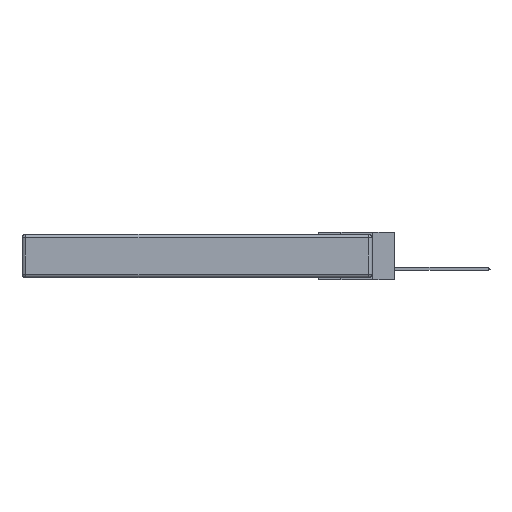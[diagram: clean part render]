
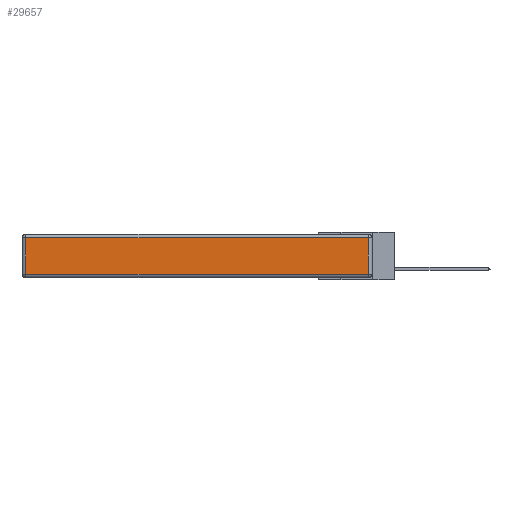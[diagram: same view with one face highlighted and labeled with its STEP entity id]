
A CAD part, left-side view. The second image highlights one B-rep face of the part: STEP entity #29657.
In plain terms, the highlighted planar face has unit normal (-1, 0, 0).
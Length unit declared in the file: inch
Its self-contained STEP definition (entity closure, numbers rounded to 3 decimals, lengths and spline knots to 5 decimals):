
#355 = ORIENTED_EDGE ( 'NONE', *, *, #27498, .T. ) ;
#1030 = FACE_OUTER_BOUND ( 'NONE', #28747, .T. ) ;
#1321 = CARTESIAN_POINT ( 'NONE',  ( 0., 0., -0.313 ) ) ;
#1453 = DIRECTION ( 'NONE',  ( -1., 0., 0. ) ) ;
#3371 = AXIS2_PLACEMENT_3D ( 'NONE', #3744, #1453, #3853 ) ;
#3744 = CARTESIAN_POINT ( 'NONE',  ( 0., 0., -0.343 ) ) ;
#3853 = DIRECTION ( 'NONE',  ( 0., 0., 1. ) ) ;
#5973 = CARTESIAN_POINT ( 'NONE',  ( 0., 0.03, -0.03 ) ) ;
#7450 = VERTEX_POINT ( 'NONE', #26897 ) ;
#8396 = VERTEX_POINT ( 'NONE', #5973 ) ;
#8527 = DIRECTION ( 'NONE',  ( 0., -1., 0. ) ) ;
#8726 = VERTEX_POINT ( 'NONE', #10129 ) ;
#9781 = LINE ( 'NONE', #1321, #25266 ) ;
#10129 = CARTESIAN_POINT ( 'NONE',  ( 0., 0.03, -0.313 ) ) ;
#10748 = CARTESIAN_POINT ( 'NONE',  ( 0., 2.72, -0.343 ) ) ;
#10846 = LINE ( 'NONE', #10748, #16578 ) ;
#12930 = PLANE ( 'NONE',  #3371 ) ;
#13310 = LINE ( 'NONE', #17860, #27780 ) ;
#15014 = ORIENTED_EDGE ( 'NONE', *, *, #17066, .T. ) ;
#15213 = CARTESIAN_POINT ( 'NONE',  ( 0., 2.72, -0.313 ) ) ;
#16578 = VECTOR ( 'NONE', #29618, 39.37008 ) ;
#17066 = EDGE_CURVE ( 'NONE', #7450, #24950, #10846, .T. ) ;
#17439 = ORIENTED_EDGE ( 'NONE', *, *, #23366, .T. ) ;
#17860 = CARTESIAN_POINT ( 'NONE',  ( 0., 0.03, -0.343 ) ) ;
#19138 = VECTOR ( 'NONE', #21898, 39.37008 ) ;
#19484 = LINE ( 'NONE', #28806, #19138 ) ;
#20246 = ORIENTED_EDGE ( 'NONE', *, *, #26650, .T. ) ;
#21898 = DIRECTION ( 'NONE',  ( 0., 1., 0. ) ) ;
#23366 = EDGE_CURVE ( 'NONE', #24950, #8726, #9781, .T. ) ;
#24950 = VERTEX_POINT ( 'NONE', #15213 ) ;
#25266 = VECTOR ( 'NONE', #8527, 39.37008 ) ;
#26650 = EDGE_CURVE ( 'NONE', #8396, #7450, #19484, .T. ) ;
#26897 = CARTESIAN_POINT ( 'NONE',  ( 0., 2.72, -0.03 ) ) ;
#27438 = DIRECTION ( 'NONE',  ( 0., 0., 1. ) ) ;
#27498 = EDGE_CURVE ( 'NONE', #8726, #8396, #13310, .T. ) ;
#27780 = VECTOR ( 'NONE', #27438, 39.37008 ) ;
#28747 = EDGE_LOOP ( 'NONE', ( #17439, #355, #20246, #15014 ) ) ;
#28806 = CARTESIAN_POINT ( 'NONE',  ( 0., 2.75, -0.03 ) ) ;
#29618 = DIRECTION ( 'NONE',  ( 0., 0., -1. ) ) ;
#29657 = ADVANCED_FACE ( 'NONE', ( #1030 ), #12930, .T. ) ;
